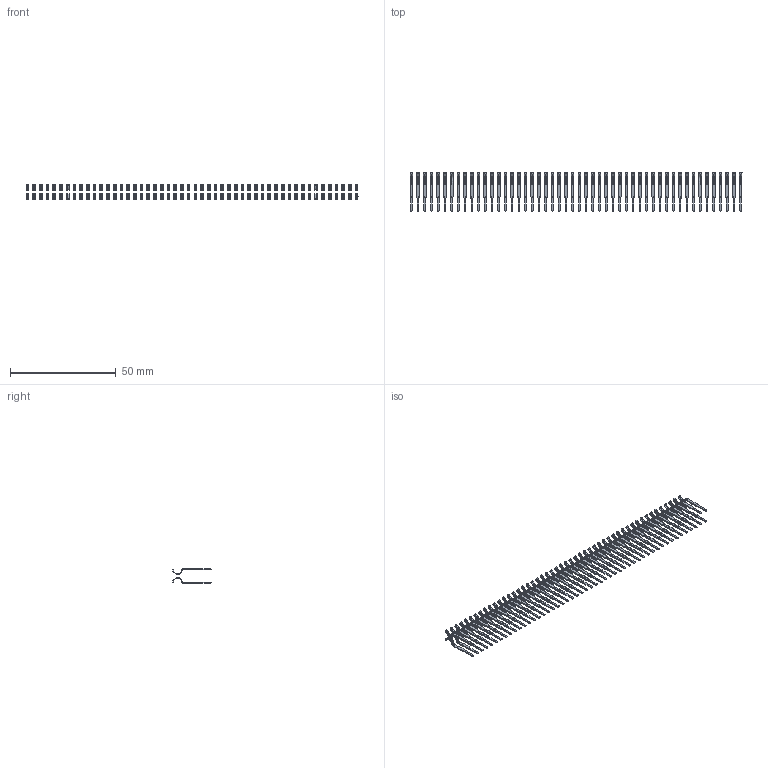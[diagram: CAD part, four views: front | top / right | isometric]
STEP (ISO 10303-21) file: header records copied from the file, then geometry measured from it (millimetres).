
FILE_DESCRIPTION (( 'STEP AP203' ), '1' );
FILE_NAME ('346-100-520-802.STEP', '2018-08-30T10:14:24', ( '' ), ( '' ), 'SwSTEP 2.0', 'SolidWorks 2016', '' );
FILE_SCHEMA (( 'CONFIG_CONTROL_DESIGN' ));
Length unit declared in the file: inch
Products named in the file (3): 346 Part_0.170 Offset - 0.128 Dia; 345-292-001_345-293-120; 346-100-520-802
Assembly tree (101 placements, depth 2):
  346-100-520-802
    346 Part_0.170 Offset - 0.128 Dia
    345-292-001_345-293-120  x100
Bounding box: 156.84 x 18.11 x 6.99 mm (x, y, z)
Volume: 855.8 mm3; surface area: 6263.1 mm2
Topology: 100 solids, 100 shells, 5000 faces, 14200 edges, 9200 vertices
Faces by surface type: plane 3200, cylinder 1800
Entity records: 31803 total; most frequent: CARTESIAN_POINT 5244, ORIENTED_EDGE 5166, DIRECTION 4659, EDGE_CURVE 2583, VECTOR 2247, LINE 2247, VERTEX_POINT 1718, AXIS2_PLACEMENT_3D 1206
